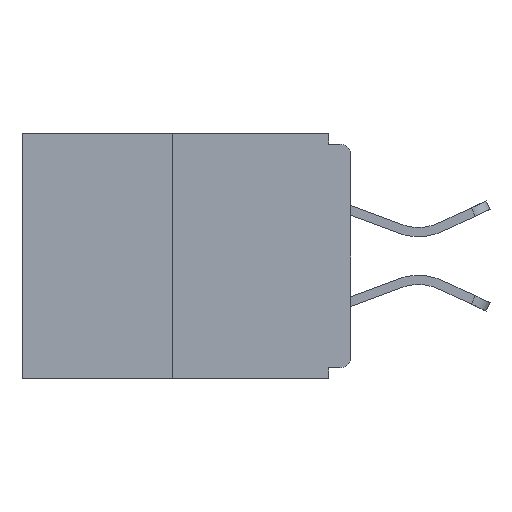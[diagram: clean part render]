
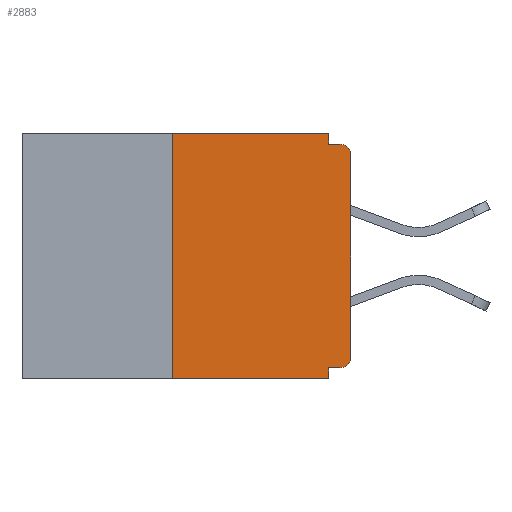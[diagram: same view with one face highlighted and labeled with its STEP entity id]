
A CAD part, left-side view. The second image highlights one B-rep face of the part: STEP entity #2883.
In plain terms, the highlighted planar face has unit normal (-1, 0, 0).
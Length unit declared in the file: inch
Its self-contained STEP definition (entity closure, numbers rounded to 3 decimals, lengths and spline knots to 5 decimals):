
#113 = DIRECTION ( 'NONE',  ( 0., 0., -1. ) ) ;
#119 = VERTEX_POINT ( 'NONE', #8677 ) ;
#187 = AXIS2_PLACEMENT_3D ( 'NONE', #17273, #11226, #113 ) ;
#257 = LINE ( 'NONE', #18509, #16586 ) ;
#1000 = DIRECTION ( 'NONE',  ( 0., -1., 0. ) ) ;
#1892 = VECTOR ( 'NONE', #1000, 39.37008 ) ;
#2546 = VERTEX_POINT ( 'NONE', #13423 ) ;
#2719 = VECTOR ( 'NONE', #6945, 39.37008 ) ;
#2883 = ADVANCED_FACE ( 'NONE', ( #18985 ), #5362, .F. ) ;
#2990 = DIRECTION ( 'NONE',  ( 0., 0., -1. ) ) ;
#3306 = AXIS2_PLACEMENT_3D ( 'NONE', #4393, #15286, #16902 ) ;
#3364 = ORIENTED_EDGE ( 'NONE', *, *, #7069, .T. ) ;
#3424 = ORIENTED_EDGE ( 'NONE', *, *, #13111, .F. ) ;
#3705 = VERTEX_POINT ( 'NONE', #6118 ) ;
#3716 = EDGE_CURVE ( 'NONE', #9947, #17437, #257, .T. ) ;
#3898 = ORIENTED_EDGE ( 'NONE', *, *, #3716, .F. ) ;
#4302 = ORIENTED_EDGE ( 'NONE', *, *, #8257, .T. ) ;
#4316 = ORIENTED_EDGE ( 'NONE', *, *, #13085, .F. ) ;
#4393 = CARTESIAN_POINT ( 'NONE',  ( 0., 0.015, -0.03 ) ) ;
#5362 = PLANE ( 'NONE',  #8979 ) ;
#5483 = VERTEX_POINT ( 'NONE', #12565 ) ;
#5562 = DIRECTION ( 'NONE',  ( 1., 0., 0. ) ) ;
#5729 = VECTOR ( 'NONE', #18533, 39.37008 ) ;
#6118 = CARTESIAN_POINT ( 'NONE',  ( 0., 0.015, -0.015 ) ) ;
#6128 = LINE ( 'NONE', #9168, #17552 ) ;
#6945 = DIRECTION ( 'NONE',  ( 0., 0., 1. ) ) ;
#7069 = EDGE_CURVE ( 'NONE', #2546, #16325, #11574, .T. ) ;
#7280 = VERTEX_POINT ( 'NONE', #14648 ) ;
#7482 = CARTESIAN_POINT ( 'NONE',  ( 0., 0.46, -0.343 ) ) ;
#7685 = CIRCLE ( 'NONE', #3306, 0.015 ) ;
#8086 = CARTESIAN_POINT ( 'NONE',  ( 0., 0.25, 0. ) ) ;
#8163 = CARTESIAN_POINT ( 'NONE',  ( 0., 0.031, -0.343 ) ) ;
#8257 = EDGE_CURVE ( 'NONE', #5483, #3705, #7685, .T. ) ;
#8647 = CARTESIAN_POINT ( 'NONE',  ( 0., 0.46, 0. ) ) ;
#8677 = CARTESIAN_POINT ( 'NONE',  ( 0., 0.25, 0. ) ) ;
#8808 = DIRECTION ( 'NONE',  ( 0., -1., 0. ) ) ;
#8979 = AXIS2_PLACEMENT_3D ( 'NONE', #8647, #5562, #19514 ) ;
#8993 = ORIENTED_EDGE ( 'NONE', *, *, #9713, .F. ) ;
#9167 = ORIENTED_EDGE ( 'NONE', *, *, #10520, .T. ) ;
#9168 = CARTESIAN_POINT ( 'NONE',  ( 0., 0., 0. ) ) ;
#9713 = EDGE_CURVE ( 'NONE', #7280, #18484, #13909, .T. ) ;
#9947 = VERTEX_POINT ( 'NONE', #13881 ) ;
#10520 = EDGE_CURVE ( 'NONE', #7280, #18272, #14668, .T. ) ;
#10901 = LINE ( 'NONE', #13481, #1892 ) ;
#10958 = EDGE_CURVE ( 'NONE', #18272, #5483, #6128, .T. ) ;
#10991 = VECTOR ( 'NONE', #14259, 39.37008 ) ;
#11127 = CARTESIAN_POINT ( 'NONE',  ( 0., 0.031, -0.343 ) ) ;
#11226 = DIRECTION ( 'NONE',  ( -1., 0., 0. ) ) ;
#11228 = EDGE_CURVE ( 'NONE', #18484, #16325, #12665, .T. ) ;
#11405 = ORIENTED_EDGE ( 'NONE', *, *, #16294, .F. ) ;
#11574 = LINE ( 'NONE', #7482, #5729 ) ;
#11758 = LINE ( 'NONE', #8086, #2719 ) ;
#12565 = CARTESIAN_POINT ( 'NONE',  ( 0., 0., -0.03 ) ) ;
#12665 = LINE ( 'NONE', #11127, #10991 ) ;
#13085 = EDGE_CURVE ( 'NONE', #119, #9947, #10901, .T. ) ;
#13111 = EDGE_CURVE ( 'NONE', #17437, #3705, #16981, .T. ) ;
#13423 = CARTESIAN_POINT ( 'NONE',  ( 0., 0.25, -0.343 ) ) ;
#13438 = CARTESIAN_POINT ( 'NONE',  ( 0., 0.031, -0.328 ) ) ;
#13481 = CARTESIAN_POINT ( 'NONE',  ( 0., 0.46, 0. ) ) ;
#13881 = CARTESIAN_POINT ( 'NONE',  ( 0., 0.031, 0. ) ) ;
#13909 = LINE ( 'NONE', #19780, #18301 ) ;
#14259 = DIRECTION ( 'NONE',  ( 0., 0., -1. ) ) ;
#14648 = CARTESIAN_POINT ( 'NONE',  ( 0., 0.015, -0.328 ) ) ;
#14668 = CIRCLE ( 'NONE', #187, 0.015 ) ;
#14799 = CARTESIAN_POINT ( 'NONE',  ( 0., 0., -0.313 ) ) ;
#15286 = DIRECTION ( 'NONE',  ( -1., 0., 0. ) ) ;
#16294 = EDGE_CURVE ( 'NONE', #2546, #119, #11758, .T. ) ;
#16319 = EDGE_LOOP ( 'NONE', ( #4316, #11405, #3364, #18687, #8993, #9167, #18667, #4302, #3424, #3898 ) ) ;
#16325 = VERTEX_POINT ( 'NONE', #8163 ) ;
#16586 = VECTOR ( 'NONE', #2990, 39.37008 ) ;
#16774 = DIRECTION ( 'NONE',  ( 0., 0., 1. ) ) ;
#16902 = DIRECTION ( 'NONE',  ( 0., 0., -1. ) ) ;
#16981 = LINE ( 'NONE', #18108, #17963 ) ;
#17273 = CARTESIAN_POINT ( 'NONE',  ( 0., 0.015, -0.313 ) ) ;
#17437 = VERTEX_POINT ( 'NONE', #18929 ) ;
#17552 = VECTOR ( 'NONE', #16774, 39.37008 ) ;
#17963 = VECTOR ( 'NONE', #8808, 39.37008 ) ;
#18108 = CARTESIAN_POINT ( 'NONE',  ( 0., 0., -0.015 ) ) ;
#18272 = VERTEX_POINT ( 'NONE', #14799 ) ;
#18301 = VECTOR ( 'NONE', #18430, 39.37008 ) ;
#18430 = DIRECTION ( 'NONE',  ( 0., 1., 0. ) ) ;
#18484 = VERTEX_POINT ( 'NONE', #13438 ) ;
#18509 = CARTESIAN_POINT ( 'NONE',  ( 0., 0.031, 0. ) ) ;
#18533 = DIRECTION ( 'NONE',  ( 0., -1., 0. ) ) ;
#18667 = ORIENTED_EDGE ( 'NONE', *, *, #10958, .T. ) ;
#18687 = ORIENTED_EDGE ( 'NONE', *, *, #11228, .F. ) ;
#18929 = CARTESIAN_POINT ( 'NONE',  ( 0., 0.031, -0.015 ) ) ;
#18985 = FACE_OUTER_BOUND ( 'NONE', #16319, .T. ) ;
#19514 = DIRECTION ( 'NONE',  ( 0., 0., -1. ) ) ;
#19780 = CARTESIAN_POINT ( 'NONE',  ( 0., 0., -0.328 ) ) ;
